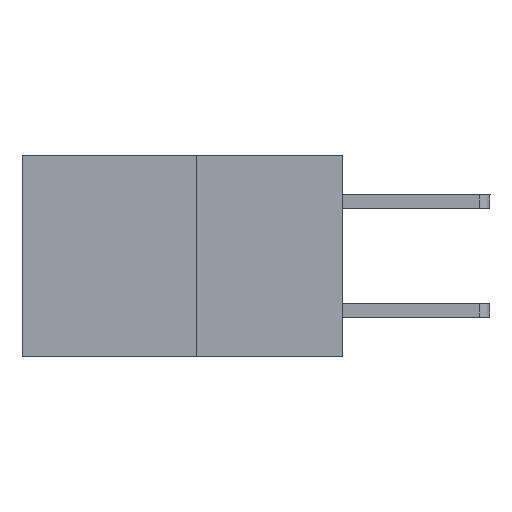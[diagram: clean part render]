
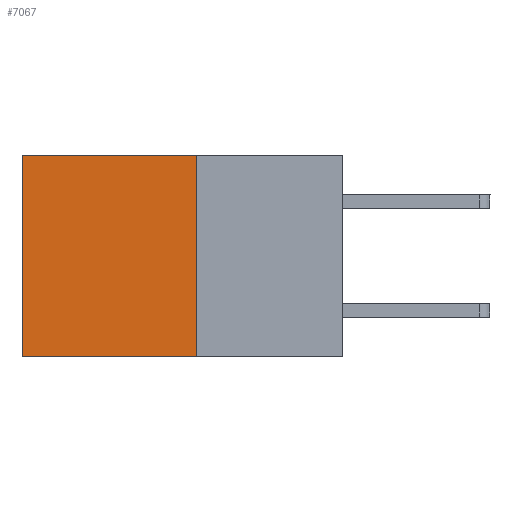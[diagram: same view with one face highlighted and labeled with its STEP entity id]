
A CAD part, left-side view. The second image highlights one B-rep face of the part: STEP entity #7067.
In plain terms, the highlighted planar face has unit normal (-1, 0, 0).
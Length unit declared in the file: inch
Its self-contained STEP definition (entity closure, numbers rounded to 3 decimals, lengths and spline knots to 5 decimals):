
#172 = VECTOR ( 'NONE', #5691, 39.37008 ) ;
#220 = CARTESIAN_POINT ( 'NONE',  ( 0.277, 0.59, -0.37 ) ) ;
#613 = VERTEX_POINT ( 'NONE', #5259 ) ;
#721 = EDGE_LOOP ( 'NONE', ( #3794, #5876, #8639, #1258 ) ) ;
#765 = EDGE_CURVE ( 'NONE', #613, #4257, #4777, .T. ) ;
#1079 = CARTESIAN_POINT ( 'NONE',  ( 0.277, 0.27, -0.37 ) ) ;
#1242 = EDGE_CURVE ( 'NONE', #7106, #8555, #6777, .T. ) ;
#1258 = ORIENTED_EDGE ( 'NONE', *, *, #1637, .T. ) ;
#1286 = DIRECTION ( 'NONE',  ( 0., 0., -1. ) ) ;
#1582 = LINE ( 'NONE', #2846, #172 ) ;
#1637 = EDGE_CURVE ( 'NONE', #613, #7106, #5254, .T. ) ;
#2846 = CARTESIAN_POINT ( 'NONE',  ( 0.277, 0.27, -0.37 ) ) ;
#2854 = CARTESIAN_POINT ( 'NONE',  ( 0.277, 0.59, 0. ) ) ;
#3225 = CARTESIAN_POINT ( 'NONE',  ( 0.277, 0.59, -0.37 ) ) ;
#3441 = CARTESIAN_POINT ( 'NONE',  ( 0.277, 0.27, -0.37 ) ) ;
#3794 = ORIENTED_EDGE ( 'NONE', *, *, #1242, .T. ) ;
#3825 = DIRECTION ( 'NONE',  ( 0., 0., -1. ) ) ;
#3983 = DIRECTION ( 'NONE',  ( 1., 0., 0. ) ) ;
#4017 = DIRECTION ( 'NONE',  ( 0., 0., -1. ) ) ;
#4257 = VERTEX_POINT ( 'NONE', #4726 ) ;
#4726 = CARTESIAN_POINT ( 'NONE',  ( 0.277, 0.27, -0.37 ) ) ;
#4777 = LINE ( 'NONE', #3441, #8611 ) ;
#5145 = VECTOR ( 'NONE', #4017, 39.37008 ) ;
#5254 = LINE ( 'NONE', #5379, #8801 ) ;
#5259 = CARTESIAN_POINT ( 'NONE',  ( 0.277, 0.27, 0. ) ) ;
#5379 = CARTESIAN_POINT ( 'NONE',  ( 0.277, 0.27, 0. ) ) ;
#5691 = DIRECTION ( 'NONE',  ( 0., 1., 0. ) ) ;
#5876 = ORIENTED_EDGE ( 'NONE', *, *, #7711, .F. ) ;
#6330 = AXIS2_PLACEMENT_3D ( 'NONE', #1079, #3983, #3825 ) ;
#6777 = LINE ( 'NONE', #3225, #5145 ) ;
#7067 = ADVANCED_FACE ( 'NONE', ( #7213 ), #7381, .F. ) ;
#7106 = VERTEX_POINT ( 'NONE', #2854 ) ;
#7213 = FACE_OUTER_BOUND ( 'NONE', #721, .T. ) ;
#7381 = PLANE ( 'NONE',  #6330 ) ;
#7711 = EDGE_CURVE ( 'NONE', #4257, #8555, #1582, .T. ) ;
#7992 = DIRECTION ( 'NONE',  ( 0., 1., 0. ) ) ;
#8555 = VERTEX_POINT ( 'NONE', #220 ) ;
#8611 = VECTOR ( 'NONE', #1286, 39.37008 ) ;
#8639 = ORIENTED_EDGE ( 'NONE', *, *, #765, .F. ) ;
#8801 = VECTOR ( 'NONE', #7992, 39.37008 ) ;
